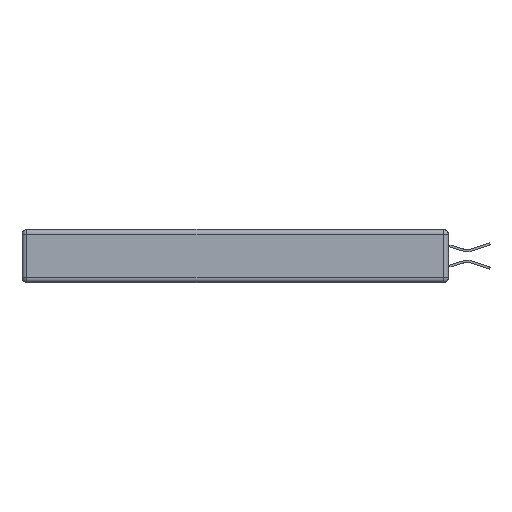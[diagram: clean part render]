
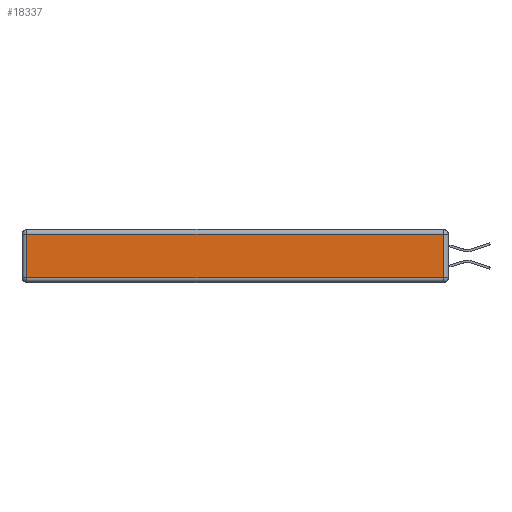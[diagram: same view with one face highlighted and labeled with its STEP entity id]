
A CAD part, left-side view. The second image highlights one B-rep face of the part: STEP entity #18337.
In plain terms, the highlighted planar face has unit normal (-1, 0, 0).
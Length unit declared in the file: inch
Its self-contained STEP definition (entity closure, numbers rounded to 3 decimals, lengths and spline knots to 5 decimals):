
#768 = ORIENTED_EDGE ( 'NONE', *, *, #13356, .T. ) ;
#1599 = EDGE_CURVE ( 'NONE', #3420, #18524, #11043, .T. ) ;
#1861 = EDGE_LOOP ( 'NONE', ( #4164, #5756, #768, #11545 ) ) ;
#2128 = VERTEX_POINT ( 'NONE', #18191 ) ;
#2492 = DIRECTION ( 'NONE',  ( -1., 0., 0. ) ) ;
#2914 = DIRECTION ( 'NONE',  ( 0., 1., 0. ) ) ;
#3420 = VERTEX_POINT ( 'NONE', #25598 ) ;
#4164 = ORIENTED_EDGE ( 'NONE', *, *, #11671, .T. ) ;
#4838 = CARTESIAN_POINT ( 'NONE',  ( 0., 2.72, -0.343 ) ) ;
#4842 = CARTESIAN_POINT ( 'NONE',  ( 0., 0.03, -0.343 ) ) ;
#4923 = CARTESIAN_POINT ( 'NONE',  ( 0., 2.75, -0.03 ) ) ;
#5570 = DIRECTION ( 'NONE',  ( 0., -1., 0. ) ) ;
#5756 = ORIENTED_EDGE ( 'NONE', *, *, #13466, .T. ) ;
#5898 = VERTEX_POINT ( 'NONE', #12273 ) ;
#6005 = LINE ( 'NONE', #4923, #13388 ) ;
#6202 = FACE_OUTER_BOUND ( 'NONE', #1861, .T. ) ;
#6396 = AXIS2_PLACEMENT_3D ( 'NONE', #16963, #2492, #6477 ) ;
#6477 = DIRECTION ( 'NONE',  ( 0., 0., 1. ) ) ;
#6993 = DIRECTION ( 'NONE',  ( 0., 0., 1. ) ) ;
#8979 = DIRECTION ( 'NONE',  ( 0., 0., -1. ) ) ;
#11043 = LINE ( 'NONE', #4838, #11661 ) ;
#11156 = CARTESIAN_POINT ( 'NONE',  ( 0., 0., -0.313 ) ) ;
#11545 = ORIENTED_EDGE ( 'NONE', *, *, #1599, .T. ) ;
#11661 = VECTOR ( 'NONE', #8979, 39.37008 ) ;
#11671 = EDGE_CURVE ( 'NONE', #18524, #5898, #20595, .T. ) ;
#12085 = VECTOR ( 'NONE', #6993, 39.37008 ) ;
#12273 = CARTESIAN_POINT ( 'NONE',  ( 0., 0.03, -0.313 ) ) ;
#12765 = LINE ( 'NONE', #4842, #12085 ) ;
#13356 = EDGE_CURVE ( 'NONE', #2128, #3420, #6005, .T. ) ;
#13388 = VECTOR ( 'NONE', #2914, 39.37008 ) ;
#13466 = EDGE_CURVE ( 'NONE', #5898, #2128, #12765, .T. ) ;
#13782 = VECTOR ( 'NONE', #5570, 39.37008 ) ;
#15096 = CARTESIAN_POINT ( 'NONE',  ( 0., 2.72, -0.313 ) ) ;
#16790 = PLANE ( 'NONE',  #6396 ) ;
#16963 = CARTESIAN_POINT ( 'NONE',  ( 0., 0., -0.343 ) ) ;
#18191 = CARTESIAN_POINT ( 'NONE',  ( 0., 0.03, -0.03 ) ) ;
#18337 = ADVANCED_FACE ( 'NONE', ( #6202 ), #16790, .T. ) ;
#18524 = VERTEX_POINT ( 'NONE', #15096 ) ;
#20595 = LINE ( 'NONE', #11156, #13782 ) ;
#25598 = CARTESIAN_POINT ( 'NONE',  ( 0., 2.72, -0.03 ) ) ;
